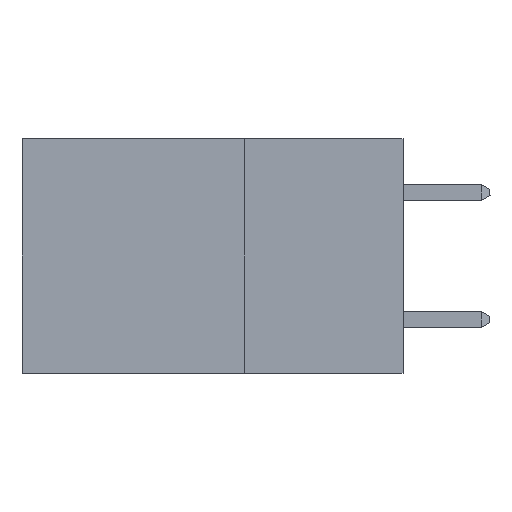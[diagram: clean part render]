
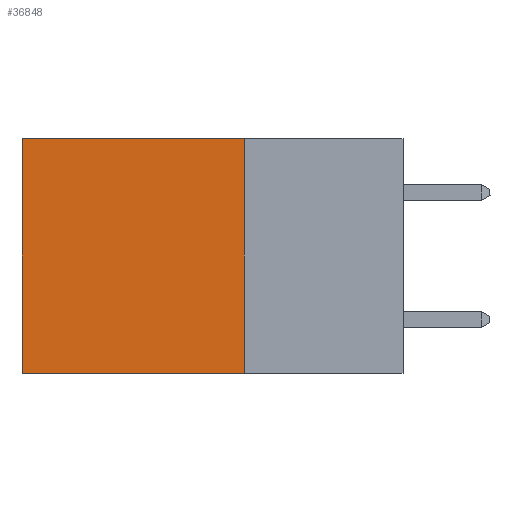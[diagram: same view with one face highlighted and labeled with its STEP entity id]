
A CAD part, left-side view. The second image highlights one B-rep face of the part: STEP entity #36848.
In plain terms, the highlighted planar face has unit normal (-1, 0, 0).
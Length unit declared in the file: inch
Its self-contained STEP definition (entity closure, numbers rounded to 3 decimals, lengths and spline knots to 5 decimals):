
#1601 = VECTOR ( 'NONE', #19816, 39.37008 ) ;
#2381 = VERTEX_POINT ( 'NONE', #12448 ) ;
#5061 = CARTESIAN_POINT ( 'NONE',  ( 0.2875, 0.25, 0. ) ) ;
#5485 = ORIENTED_EDGE ( 'NONE', *, *, #10024, .F. ) ;
#5972 = FACE_OUTER_BOUND ( 'NONE', #15149, .T. ) ;
#6374 = DIRECTION ( 'NONE',  ( 0., 1., 0. ) ) ;
#6759 = ORIENTED_EDGE ( 'NONE', *, *, #16822, .F. ) ;
#10024 = EDGE_CURVE ( 'NONE', #26611, #26916, #13759, .T. ) ;
#10850 = VECTOR ( 'NONE', #27179, 39.37008 ) ;
#11633 = CARTESIAN_POINT ( 'NONE',  ( 0.2875, 0.25, -0.37 ) ) ;
#11970 = AXIS2_PLACEMENT_3D ( 'NONE', #18890, #12809, #37281 ) ;
#12448 = CARTESIAN_POINT ( 'NONE',  ( 0.2875, 0.6, -0.37 ) ) ;
#12809 = DIRECTION ( 'NONE',  ( 1., 0., 0. ) ) ;
#13019 = PLANE ( 'NONE',  #11970 ) ;
#13022 = VECTOR ( 'NONE', #6374, 39.37008 ) ;
#13160 = EDGE_CURVE ( 'NONE', #16849, #2381, #24526, .T. ) ;
#13759 = LINE ( 'NONE', #5061, #1601 ) ;
#15149 = EDGE_LOOP ( 'NONE', ( #24525, #6759, #5485, #35220 ) ) ;
#16822 = EDGE_CURVE ( 'NONE', #26916, #2381, #27015, .T. ) ;
#16849 = VERTEX_POINT ( 'NONE', #32696 ) ;
#17139 = EDGE_CURVE ( 'NONE', #26611, #16849, #18502, .T. ) ;
#17538 = VECTOR ( 'NONE', #23979, 39.37008 ) ;
#17689 = CARTESIAN_POINT ( 'NONE',  ( 0.2875, 0.25, -0.37 ) ) ;
#18502 = LINE ( 'NONE', #30845, #13022 ) ;
#18890 = CARTESIAN_POINT ( 'NONE',  ( 0.2875, 0.25, 0. ) ) ;
#19816 = DIRECTION ( 'NONE',  ( 0., 0., -1. ) ) ;
#21690 = CARTESIAN_POINT ( 'NONE',  ( 0.2875, 0.6, 0. ) ) ;
#23979 = DIRECTION ( 'NONE',  ( 0., 1., 0. ) ) ;
#24525 = ORIENTED_EDGE ( 'NONE', *, *, #13160, .T. ) ;
#24526 = LINE ( 'NONE', #21690, #10850 ) ;
#24776 = CARTESIAN_POINT ( 'NONE',  ( 0.2875, 0.25, 0. ) ) ;
#26611 = VERTEX_POINT ( 'NONE', #24776 ) ;
#26916 = VERTEX_POINT ( 'NONE', #17689 ) ;
#27015 = LINE ( 'NONE', #11633, #17538 ) ;
#27179 = DIRECTION ( 'NONE',  ( 0., 0., -1. ) ) ;
#30845 = CARTESIAN_POINT ( 'NONE',  ( 0.2875, 0.25, 0. ) ) ;
#32696 = CARTESIAN_POINT ( 'NONE',  ( 0.2875, 0.6, 0. ) ) ;
#35220 = ORIENTED_EDGE ( 'NONE', *, *, #17139, .T. ) ;
#36848 = ADVANCED_FACE ( 'NONE', ( #5972 ), #13019, .F. ) ;
#37281 = DIRECTION ( 'NONE',  ( 0., 0., -1. ) ) ;
